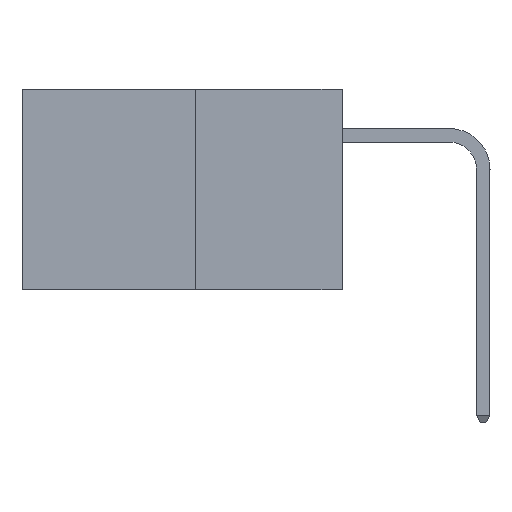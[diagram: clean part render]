
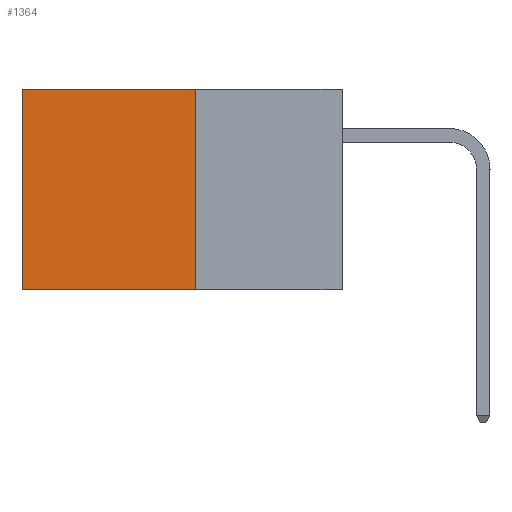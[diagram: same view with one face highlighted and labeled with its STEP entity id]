
A CAD part, left-side view. The second image highlights one B-rep face of the part: STEP entity #1364.
In plain terms, the highlighted planar face has unit normal (-1, 0, 0).
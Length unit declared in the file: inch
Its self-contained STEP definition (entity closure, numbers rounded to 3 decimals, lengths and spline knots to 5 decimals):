
#34 = EDGE_CURVE ( 'NONE', #6828, #8321, #5921, .T. ) ;
#289 = LINE ( 'NONE', #6865, #5121 ) ;
#461 = ORIENTED_EDGE ( 'NONE', *, *, #8248, .F. ) ;
#583 = LINE ( 'NONE', #9602, #7563 ) ;
#697 = EDGE_CURVE ( 'NONE', #1117, #8321, #583, .T. ) ;
#1117 = VERTEX_POINT ( 'NONE', #7577 ) ;
#1361 = CARTESIAN_POINT ( 'NONE',  ( 0.277, 0.27, -0.37 ) ) ;
#1364 = ADVANCED_FACE ( 'NONE', ( #3238 ), #4597, .F. ) ;
#1905 = DIRECTION ( 'NONE',  ( 0., 0., -1. ) ) ;
#2740 = CARTESIAN_POINT ( 'NONE',  ( 0.277, 0.27, 0. ) ) ;
#3051 = ORIENTED_EDGE ( 'NONE', *, *, #10489, .T. ) ;
#3238 = FACE_OUTER_BOUND ( 'NONE', #4713, .T. ) ;
#3657 = DIRECTION ( 'NONE',  ( 0., 0., -1. ) ) ;
#3692 = VECTOR ( 'NONE', #6405, 39.37008 ) ;
#4587 = AXIS2_PLACEMENT_3D ( 'NONE', #8134, #5064, #3657 ) ;
#4597 = PLANE ( 'NONE',  #4587 ) ;
#4713 = EDGE_LOOP ( 'NONE', ( #9007, #7213, #461, #3051 ) ) ;
#5064 = DIRECTION ( 'NONE',  ( 1., 0., 0. ) ) ;
#5121 = VECTOR ( 'NONE', #9183, 39.37008 ) ;
#5921 = LINE ( 'NONE', #1361, #3692 ) ;
#6405 = DIRECTION ( 'NONE',  ( 0., 1., 0. ) ) ;
#6828 = VERTEX_POINT ( 'NONE', #7385 ) ;
#6865 = CARTESIAN_POINT ( 'NONE',  ( 0.277, 0.27, 0. ) ) ;
#7213 = ORIENTED_EDGE ( 'NONE', *, *, #34, .F. ) ;
#7385 = CARTESIAN_POINT ( 'NONE',  ( 0.277, 0.27, -0.37 ) ) ;
#7563 = VECTOR ( 'NONE', #1905, 39.37008 ) ;
#7577 = CARTESIAN_POINT ( 'NONE',  ( 0.277, 0.59, 0. ) ) ;
#7738 = LINE ( 'NONE', #8562, #9508 ) ;
#8134 = CARTESIAN_POINT ( 'NONE',  ( 0.277, 0.27, -0.37 ) ) ;
#8248 = EDGE_CURVE ( 'NONE', #10567, #6828, #7738, .T. ) ;
#8321 = VERTEX_POINT ( 'NONE', #10123 ) ;
#8562 = CARTESIAN_POINT ( 'NONE',  ( 0.277, 0.27, -0.37 ) ) ;
#9007 = ORIENTED_EDGE ( 'NONE', *, *, #697, .T. ) ;
#9183 = DIRECTION ( 'NONE',  ( 0., 1., 0. ) ) ;
#9338 = DIRECTION ( 'NONE',  ( 0., 0., -1. ) ) ;
#9508 = VECTOR ( 'NONE', #9338, 39.37008 ) ;
#9602 = CARTESIAN_POINT ( 'NONE',  ( 0.277, 0.59, -0.37 ) ) ;
#10123 = CARTESIAN_POINT ( 'NONE',  ( 0.277, 0.59, -0.37 ) ) ;
#10489 = EDGE_CURVE ( 'NONE', #10567, #1117, #289, .T. ) ;
#10567 = VERTEX_POINT ( 'NONE', #2740 ) ;
